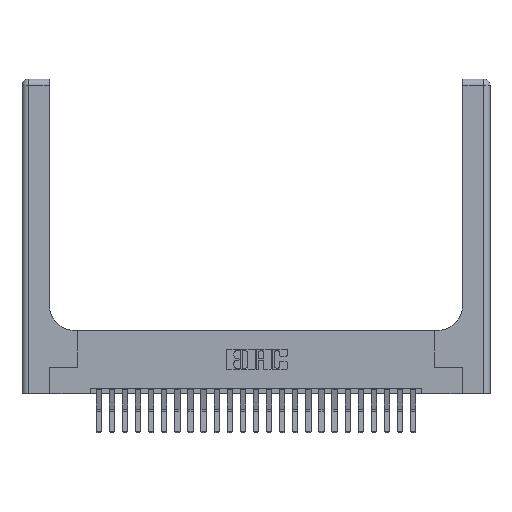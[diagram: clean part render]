
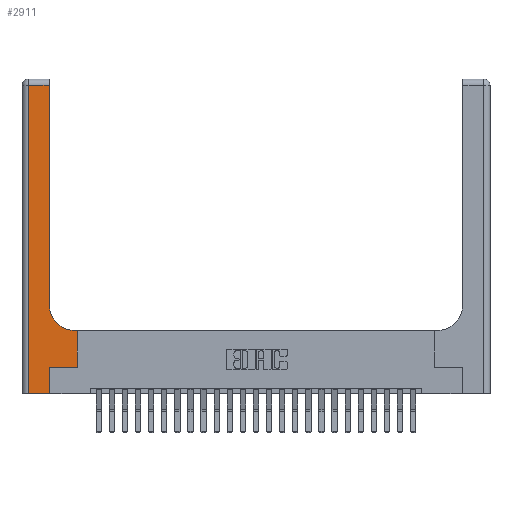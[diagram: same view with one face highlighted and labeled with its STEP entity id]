
A CAD part, top view. The second image highlights one B-rep face of the part: STEP entity #2911.
In plain terms, the highlighted planar face has unit normal (0, 0, 1).
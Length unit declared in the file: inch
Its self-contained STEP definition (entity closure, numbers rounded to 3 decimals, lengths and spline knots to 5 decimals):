
#43 = ORIENTED_EDGE ( 'NONE', *, *, #16698, .T. ) ;
#230 = AXIS2_PLACEMENT_3D ( 'NONE', #15828, #8193, #21092 ) ;
#1553 = EDGE_CURVE ( 'NONE', #15863, #21469, #13923, .T. ) ;
#1842 = LINE ( 'NONE', #22304, #20039 ) ;
#2485 = DIRECTION ( 'NONE',  ( 0., 1., 0. ) ) ;
#2911 = ADVANCED_FACE ( 'NONE', ( #10519 ), #7573, .F. ) ;
#3395 = CIRCLE ( 'NONE', #230, 0.25 ) ;
#3804 = VECTOR ( 'NONE', #15870, 39.37008 ) ;
#3812 = ORIENTED_EDGE ( 'NONE', *, *, #6581, .T. ) ;
#4904 = EDGE_CURVE ( 'NONE', #21452, #13507, #10696, .T. ) ;
#6581 = EDGE_CURVE ( 'NONE', #12807, #10972, #22742, .T. ) ;
#7573 = PLANE ( 'NONE',  #20057 ) ;
#7691 = CARTESIAN_POINT ( 'NONE',  ( 0.265, 0., 0.37 ) ) ;
#7826 = VECTOR ( 'NONE', #11252, 39.37008 ) ;
#8147 = CARTESIAN_POINT ( 'NONE',  ( 0., 2.94, 0.37 ) ) ;
#8193 = DIRECTION ( 'NONE',  ( 0., 0., -1. ) ) ;
#8287 = CARTESIAN_POINT ( 'NONE',  ( 0.528, 0.6, 0.37 ) ) ;
#8412 = VECTOR ( 'NONE', #13491, 39.37008 ) ;
#9719 = CARTESIAN_POINT ( 'NONE',  ( 0.26, 0.85, 0.37 ) ) ;
#9729 = ORIENTED_EDGE ( 'NONE', *, *, #14239, .T. ) ;
#9778 = ORIENTED_EDGE ( 'NONE', *, *, #23705, .T. ) ;
#9784 = ORIENTED_EDGE ( 'NONE', *, *, #19792, .T. ) ;
#10291 = CARTESIAN_POINT ( 'NONE',  ( 0.51, 0.6, 0.37 ) ) ;
#10519 = FACE_OUTER_BOUND ( 'NONE', #22832, .T. ) ;
#10696 = LINE ( 'NONE', #19031, #16772 ) ;
#10972 = VERTEX_POINT ( 'NONE', #10291 ) ;
#11177 = CARTESIAN_POINT ( 'NONE',  ( 0.06, 2.94, 0.37 ) ) ;
#11208 = VERTEX_POINT ( 'NONE', #15579 ) ;
#11243 = DIRECTION ( 'NONE',  ( 1., 0., 0. ) ) ;
#11252 = DIRECTION ( 'NONE',  ( 0., 1., 0. ) ) ;
#11430 = DIRECTION ( 'NONE',  ( 0., 1., 0. ) ) ;
#11643 = LINE ( 'NONE', #23615, #12800 ) ;
#11680 = CARTESIAN_POINT ( 'NONE',  ( 0.528, 0.25, 0.37 ) ) ;
#12084 = CARTESIAN_POINT ( 'NONE',  ( 0.06, 0., 0.37 ) ) ;
#12121 = LINE ( 'NONE', #22315, #7826 ) ;
#12695 = VERTEX_POINT ( 'NONE', #9719 ) ;
#12800 = VECTOR ( 'NONE', #2485, 39.37008 ) ;
#12807 = VERTEX_POINT ( 'NONE', #8287 ) ;
#12900 = VECTOR ( 'NONE', #18861, 39.37008 ) ;
#12957 = LINE ( 'NONE', #15002, #17040 ) ;
#13105 = CARTESIAN_POINT ( 'NONE',  ( 0., 3., 0.37 ) ) ;
#13491 = DIRECTION ( 'NONE',  ( -1., 0., 0. ) ) ;
#13507 = VERTEX_POINT ( 'NONE', #11680 ) ;
#13923 = LINE ( 'NONE', #15468, #3804 ) ;
#14159 = EDGE_CURVE ( 'NONE', #21230, #21452, #12121, .T. ) ;
#14239 = EDGE_CURVE ( 'NONE', #11208, #15863, #21960, .T. ) ;
#15002 = CARTESIAN_POINT ( 'NONE',  ( 0.528, 0.25, 0.37 ) ) ;
#15468 = CARTESIAN_POINT ( 'NONE',  ( 0.06, 3., 0.37 ) ) ;
#15579 = CARTESIAN_POINT ( 'NONE',  ( 0.26, 2.94, 0.37 ) ) ;
#15828 = CARTESIAN_POINT ( 'NONE',  ( 0.51, 0.85, 0.37 ) ) ;
#15863 = VERTEX_POINT ( 'NONE', #11177 ) ;
#15870 = DIRECTION ( 'NONE',  ( 0., -1., 0. ) ) ;
#16698 = EDGE_CURVE ( 'NONE', #13507, #12807, #12957, .T. ) ;
#16772 = VECTOR ( 'NONE', #22899, 39.37008 ) ;
#16773 = DIRECTION ( 'NONE',  ( -1., 0., 0. ) ) ;
#17040 = VECTOR ( 'NONE', #11430, 39.37008 ) ;
#18861 = DIRECTION ( 'NONE',  ( -1., 0., 0. ) ) ;
#19031 = CARTESIAN_POINT ( 'NONE',  ( 0.265, 0.25, 0.37 ) ) ;
#19792 = EDGE_CURVE ( 'NONE', #12695, #11208, #11643, .T. ) ;
#20039 = VECTOR ( 'NONE', #11243, 39.37008 ) ;
#20057 = AXIS2_PLACEMENT_3D ( 'NONE', #13105, #20293, #16773 ) ;
#20293 = DIRECTION ( 'NONE',  ( 0., 0., -1. ) ) ;
#20388 = ORIENTED_EDGE ( 'NONE', *, *, #4904, .T. ) ;
#20453 = EDGE_CURVE ( 'NONE', #21469, #21230, #1842, .T. ) ;
#20454 = ORIENTED_EDGE ( 'NONE', *, *, #14159, .T. ) ;
#20560 = CARTESIAN_POINT ( 'NONE',  ( 0.26, 0.6, 0.37 ) ) ;
#20675 = ORIENTED_EDGE ( 'NONE', *, *, #1553, .T. ) ;
#21092 = DIRECTION ( 'NONE',  ( 1., 0., 0. ) ) ;
#21230 = VERTEX_POINT ( 'NONE', #7691 ) ;
#21452 = VERTEX_POINT ( 'NONE', #23012 ) ;
#21469 = VERTEX_POINT ( 'NONE', #12084 ) ;
#21960 = LINE ( 'NONE', #8147, #8412 ) ;
#22304 = CARTESIAN_POINT ( 'NONE',  ( 0., 0., 0.37 ) ) ;
#22315 = CARTESIAN_POINT ( 'NONE',  ( 0.265, 0., 0.37 ) ) ;
#22335 = ORIENTED_EDGE ( 'NONE', *, *, #20453, .T. ) ;
#22742 = LINE ( 'NONE', #20560, #12900 ) ;
#22832 = EDGE_LOOP ( 'NONE', ( #9784, #9729, #20675, #22335, #20454, #20388, #43, #3812, #9778 ) ) ;
#22899 = DIRECTION ( 'NONE',  ( 1., 0., 0. ) ) ;
#23012 = CARTESIAN_POINT ( 'NONE',  ( 0.265, 0.25, 0.37 ) ) ;
#23615 = CARTESIAN_POINT ( 'NONE',  ( 0.26, 3., 0.37 ) ) ;
#23705 = EDGE_CURVE ( 'NONE', #10972, #12695, #3395, .T. ) ;
